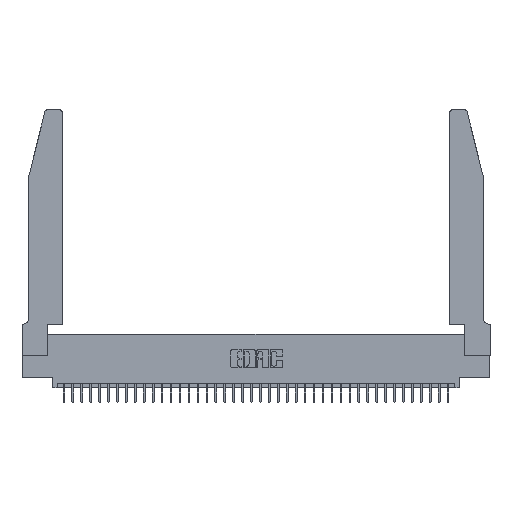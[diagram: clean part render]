
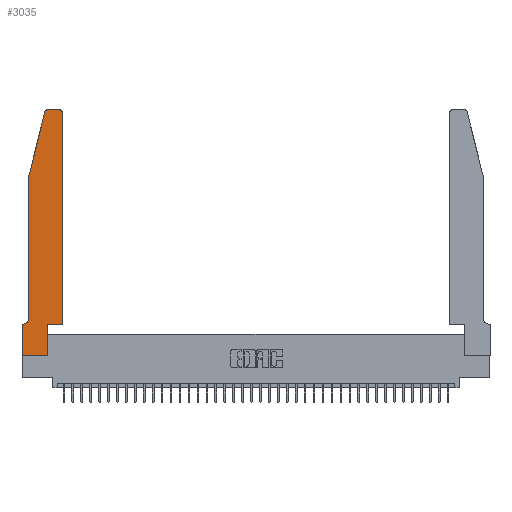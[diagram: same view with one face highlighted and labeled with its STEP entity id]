
A CAD part, top view. The second image highlights one B-rep face of the part: STEP entity #3035.
In plain terms, the highlighted planar face has unit normal (0, 0, 1).
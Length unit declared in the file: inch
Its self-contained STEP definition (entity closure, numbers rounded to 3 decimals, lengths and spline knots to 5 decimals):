
#95 = DIRECTION ( 'NONE',  ( 1., 0., 0. ) ) ;
#357 = ORIENTED_EDGE ( 'NONE', *, *, #26501, .T. ) ;
#1197 = AXIS2_PLACEMENT_3D ( 'NONE', #21410, #36493, #18533 ) ;
#2446 = CARTESIAN_POINT ( 'NONE',  ( 0.4505, 2.72, 0.37 ) ) ;
#3035 = ADVANCED_FACE ( 'NONE', ( #20471 ), #9454, .T. ) ;
#3721 = ORIENTED_EDGE ( 'NONE', *, *, #18025, .T. ) ;
#3975 = DIRECTION ( 'NONE',  ( 0., 0., -1. ) ) ;
#4170 = VERTEX_POINT ( 'NONE', #26553 ) ;
#4458 = ORIENTED_EDGE ( 'NONE', *, *, #35479, .T. ) ;
#5862 = CARTESIAN_POINT ( 'NONE',  ( 0.0755, 2., 0.37 ) ) ;
#7074 = VERTEX_POINT ( 'NONE', #25033 ) ;
#7672 = LINE ( 'NONE', #12736, #38723 ) ;
#8572 = CARTESIAN_POINT ( 'NONE',  ( 0.4505, 0.35, 0.37 ) ) ;
#9358 = VECTOR ( 'NONE', #95, 39.37008 ) ;
#9454 = PLANE ( 'NONE',  #1197 ) ;
#10056 = EDGE_CURVE ( 'NONE', #11313, #32429, #24897, .T. ) ;
#10299 = LINE ( 'NONE', #12388, #9358 ) ;
#10355 = ORIENTED_EDGE ( 'NONE', *, *, #34220, .T. ) ;
#10577 = EDGE_CURVE ( 'NONE', #13383, #7074, #32867, .T. ) ;
#11313 = VERTEX_POINT ( 'NONE', #15743 ) ;
#11468 = EDGE_LOOP ( 'NONE', ( #10355, #25852, #35288, #12287, #21774, #16194, #357, #12478, #35553, #39053, #3721, #4458 ) ) ;
#11697 = DIRECTION ( 'NONE',  ( -0.239, -0.971, 0. ) ) ;
#11763 = VERTEX_POINT ( 'NONE', #26584 ) ;
#11773 = VERTEX_POINT ( 'NONE', #2446 ) ;
#12287 = ORIENTED_EDGE ( 'NONE', *, *, #15058, .T. ) ;
#12388 = CARTESIAN_POINT ( 'NONE',  ( 0.4505, 0.35, 0.37 ) ) ;
#12478 = ORIENTED_EDGE ( 'NONE', *, *, #30222, .T. ) ;
#12511 = DIRECTION ( 'NONE',  ( 0., 0., 1. ) ) ;
#12691 = AXIS2_PLACEMENT_3D ( 'NONE', #30511, #12511, #33565 ) ;
#12736 = CARTESIAN_POINT ( 'NONE',  ( 0.2605, 2.75, 0.37 ) ) ;
#12879 = VERTEX_POINT ( 'NONE', #22727 ) ;
#13383 = VERTEX_POINT ( 'NONE', #37126 ) ;
#13498 = VECTOR ( 'NONE', #36301, 39.37008 ) ;
#14832 = CARTESIAN_POINT ( 'NONE',  ( 0.2865, 0.35, 0.37 ) ) ;
#15058 = EDGE_CURVE ( 'NONE', #26202, #11313, #19893, .T. ) ;
#15469 = AXIS2_PLACEMENT_3D ( 'NONE', #22189, #3975, #25172 ) ;
#15498 = VECTOR ( 'NONE', #20292, 39.37008 ) ;
#15537 = LINE ( 'NONE', #14832, #37617 ) ;
#15660 = DIRECTION ( 'NONE',  ( 0., 0., 1. ) ) ;
#15743 = CARTESIAN_POINT ( 'NONE',  ( 0.0755, 0.42, 0.37 ) ) ;
#16194 = ORIENTED_EDGE ( 'NONE', *, *, #28724, .T. ) ;
#17260 = DIRECTION ( 'NONE',  ( 0., -1., 0. ) ) ;
#17866 = DIRECTION ( 'NONE',  ( 0., 1., 0. ) ) ;
#18025 = EDGE_CURVE ( 'NONE', #35734, #11773, #27504, .T. ) ;
#18524 = CARTESIAN_POINT ( 'NONE',  ( 0., 0.35, 0.37 ) ) ;
#18533 = DIRECTION ( 'NONE',  ( 1., 0., 0. ) ) ;
#18646 = VECTOR ( 'NONE', #32632, 39.37008 ) ;
#18971 = VECTOR ( 'NONE', #36077, 39.37008 ) ;
#19893 = LINE ( 'NONE', #5862, #18971 ) ;
#20292 = DIRECTION ( 'NONE',  ( -1., 0., 0. ) ) ;
#20471 = FACE_OUTER_BOUND ( 'NONE', #11468, .T. ) ;
#21014 = CARTESIAN_POINT ( 'NONE',  ( 0.0055, 0.35, 0.37 ) ) ;
#21260 = CIRCLE ( 'NONE', #12691, 0.03 ) ;
#21410 = CARTESIAN_POINT ( 'NONE',  ( 0., 0.35, 0.37 ) ) ;
#21495 = LINE ( 'NONE', #33304, #13498 ) ;
#21774 = ORIENTED_EDGE ( 'NONE', *, *, #10056, .T. ) ;
#21825 = DIRECTION ( 'NONE',  ( -1., 0., 0. ) ) ;
#22189 = CARTESIAN_POINT ( 'NONE',  ( 0.0055, 0.42, 0.37 ) ) ;
#22727 = CARTESIAN_POINT ( 'NONE',  ( 0., 0., 0.37 ) ) ;
#22790 = EDGE_CURVE ( 'NONE', #31822, #35734, #10299, .T. ) ;
#24594 = VECTOR ( 'NONE', #17260, 39.37008 ) ;
#24897 = CIRCLE ( 'NONE', #15469, 0.07 ) ;
#25033 = CARTESIAN_POINT ( 'NONE',  ( 0.25487, 2.72718, 0.37 ) ) ;
#25172 = DIRECTION ( 'NONE',  ( -1., 0., 0. ) ) ;
#25436 = LINE ( 'NONE', #26649, #32492 ) ;
#25852 = ORIENTED_EDGE ( 'NONE', *, *, #10577, .T. ) ;
#26202 = VERTEX_POINT ( 'NONE', #34201 ) ;
#26501 = EDGE_CURVE ( 'NONE', #32523, #12879, #32602, .T. ) ;
#26553 = CARTESIAN_POINT ( 'NONE',  ( 0.2865, 0., 0.37 ) ) ;
#26584 = CARTESIAN_POINT ( 'NONE',  ( 0.4205, 2.75, 0.37 ) ) ;
#26649 = CARTESIAN_POINT ( 'NONE',  ( 0.0755, 2., 0.37 ) ) ;
#27179 = CARTESIAN_POINT ( 'NONE',  ( 0.2865, 0.35, 0.37 ) ) ;
#27504 = LINE ( 'NONE', #8572, #18646 ) ;
#28507 = CARTESIAN_POINT ( 'NONE',  ( 0.4505, 0.35, 0.37 ) ) ;
#28724 = EDGE_CURVE ( 'NONE', #32429, #32523, #38499, .T. ) ;
#30222 = EDGE_CURVE ( 'NONE', #12879, #4170, #21495, .T. ) ;
#30511 = CARTESIAN_POINT ( 'NONE',  ( 0.4205, 2.72, 0.37 ) ) ;
#31822 = VERTEX_POINT ( 'NONE', #27179 ) ;
#32429 = VERTEX_POINT ( 'NONE', #21014 ) ;
#32492 = VECTOR ( 'NONE', #11697, 39.37008 ) ;
#32523 = VERTEX_POINT ( 'NONE', #18524 ) ;
#32602 = LINE ( 'NONE', #35098, #24594 ) ;
#32632 = DIRECTION ( 'NONE',  ( 0., 1., 0. ) ) ;
#32867 = CIRCLE ( 'NONE', #38859, 0.03 ) ;
#33304 = CARTESIAN_POINT ( 'NONE',  ( 0., 0., 0.37 ) ) ;
#33565 = DIRECTION ( 'NONE',  ( 1., 0., 0. ) ) ;
#33671 = CARTESIAN_POINT ( 'NONE',  ( 0.284, 2.72, 0.37 ) ) ;
#34201 = CARTESIAN_POINT ( 'NONE',  ( 0.0755, 2., 0.37 ) ) ;
#34220 = EDGE_CURVE ( 'NONE', #11763, #13383, #7672, .T. ) ;
#35098 = CARTESIAN_POINT ( 'NONE',  ( 0., 0., 0.37 ) ) ;
#35288 = ORIENTED_EDGE ( 'NONE', *, *, #35992, .T. ) ;
#35479 = EDGE_CURVE ( 'NONE', #11773, #11763, #21260, .T. ) ;
#35553 = ORIENTED_EDGE ( 'NONE', *, *, #36583, .T. ) ;
#35734 = VERTEX_POINT ( 'NONE', #28507 ) ;
#35992 = EDGE_CURVE ( 'NONE', #7074, #26202, #25436, .T. ) ;
#36077 = DIRECTION ( 'NONE',  ( 0., -1., 0. ) ) ;
#36301 = DIRECTION ( 'NONE',  ( 1., 0., 0. ) ) ;
#36493 = DIRECTION ( 'NONE',  ( 0., 0., 1. ) ) ;
#36583 = EDGE_CURVE ( 'NONE', #4170, #31822, #15537, .T. ) ;
#36660 = DIRECTION ( 'NONE',  ( 1., 0., 0. ) ) ;
#37126 = CARTESIAN_POINT ( 'NONE',  ( 0.284, 2.75, 0.37 ) ) ;
#37617 = VECTOR ( 'NONE', #17866, 39.37008 ) ;
#38252 = CARTESIAN_POINT ( 'NONE',  ( 0.0755, 0.35, 0.37 ) ) ;
#38499 = LINE ( 'NONE', #38252, #15498 ) ;
#38723 = VECTOR ( 'NONE', #21825, 39.37008 ) ;
#38859 = AXIS2_PLACEMENT_3D ( 'NONE', #33671, #15660, #36660 ) ;
#39053 = ORIENTED_EDGE ( 'NONE', *, *, #22790, .T. ) ;
